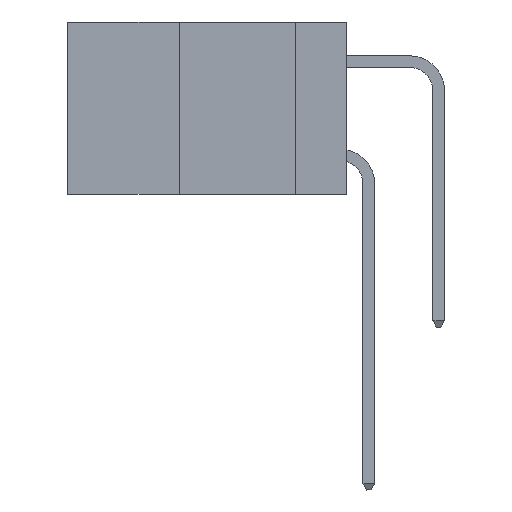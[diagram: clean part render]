
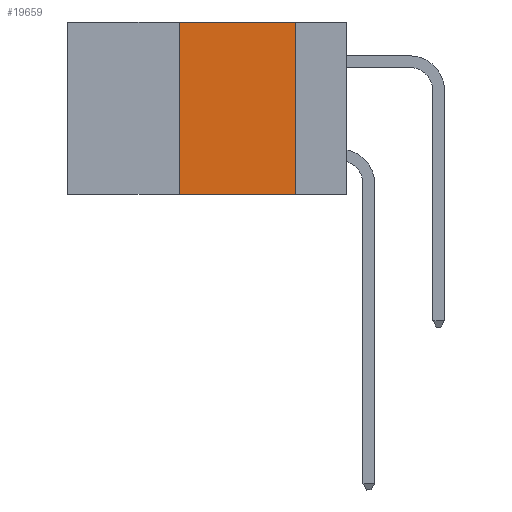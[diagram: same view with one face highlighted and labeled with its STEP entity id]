
A CAD part, left-side view. The second image highlights one B-rep face of the part: STEP entity #19659.
In plain terms, the highlighted planar face has unit normal (-1, 0, 0).
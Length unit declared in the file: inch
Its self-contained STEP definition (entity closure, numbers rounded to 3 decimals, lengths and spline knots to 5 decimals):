
#158 = CARTESIAN_POINT ( 'NONE',  ( 0., 0.36, 0. ) ) ;
#323 = AXIS2_PLACEMENT_3D ( 'NONE', #9959, #18751, #11607 ) ;
#1712 = EDGE_CURVE ( 'NONE', #13846, #12385, #18874, .T. ) ;
#2384 = DIRECTION ( 'NONE',  ( 0., -1., 0. ) ) ;
#2975 = VECTOR ( 'NONE', #18350, 39.37008 ) ;
#3906 = VECTOR ( 'NONE', #23014, 39.37008 ) ;
#4623 = CARTESIAN_POINT ( 'NONE',  ( 0., 0.11, 0. ) ) ;
#5204 = LINE ( 'NONE', #9485, #7160 ) ;
#5234 = CARTESIAN_POINT ( 'NONE',  ( 0., 0.36, -0.37 ) ) ;
#5297 = EDGE_CURVE ( 'NONE', #12617, #17508, #5204, .T. ) ;
#6290 = CARTESIAN_POINT ( 'NONE',  ( 0., 0.6, -0.37 ) ) ;
#6776 = ORIENTED_EDGE ( 'NONE', *, *, #5297, .F. ) ;
#7160 = VECTOR ( 'NONE', #2384, 39.37008 ) ;
#7684 = LINE ( 'NONE', #158, #2975 ) ;
#9485 = CARTESIAN_POINT ( 'NONE',  ( 0., 0.6, 0. ) ) ;
#9600 = DIRECTION ( 'NONE',  ( 0., -1., 0. ) ) ;
#9793 = EDGE_CURVE ( 'NONE', #17508, #12385, #22021, .T. ) ;
#9959 = CARTESIAN_POINT ( 'NONE',  ( 0., 0.6, 0. ) ) ;
#10527 = CARTESIAN_POINT ( 'NONE',  ( 0., 0.11, 0. ) ) ;
#11473 = EDGE_LOOP ( 'NONE', ( #21906, #6776, #15019, #20943 ) ) ;
#11607 = DIRECTION ( 'NONE',  ( 0., 0., -1. ) ) ;
#11686 = PLANE ( 'NONE',  #323 ) ;
#12385 = VERTEX_POINT ( 'NONE', #19049 ) ;
#12617 = VERTEX_POINT ( 'NONE', #17714 ) ;
#12756 = VECTOR ( 'NONE', #9600, 39.37008 ) ;
#13846 = VERTEX_POINT ( 'NONE', #5234 ) ;
#15019 = ORIENTED_EDGE ( 'NONE', *, *, #22614, .F. ) ;
#15377 = FACE_OUTER_BOUND ( 'NONE', #11473, .T. ) ;
#17508 = VERTEX_POINT ( 'NONE', #4623 ) ;
#17714 = CARTESIAN_POINT ( 'NONE',  ( 0., 0.36, 0. ) ) ;
#18350 = DIRECTION ( 'NONE',  ( 0., 0., 1. ) ) ;
#18751 = DIRECTION ( 'NONE',  ( 1., 0., 0. ) ) ;
#18874 = LINE ( 'NONE', #6290, #12756 ) ;
#19049 = CARTESIAN_POINT ( 'NONE',  ( 0., 0.11, -0.37 ) ) ;
#19659 = ADVANCED_FACE ( 'NONE', ( #15377 ), #11686, .F. ) ;
#20943 = ORIENTED_EDGE ( 'NONE', *, *, #1712, .T. ) ;
#21906 = ORIENTED_EDGE ( 'NONE', *, *, #9793, .F. ) ;
#22021 = LINE ( 'NONE', #10527, #3906 ) ;
#22614 = EDGE_CURVE ( 'NONE', #13846, #12617, #7684, .T. ) ;
#23014 = DIRECTION ( 'NONE',  ( 0., 0., -1. ) ) ;
